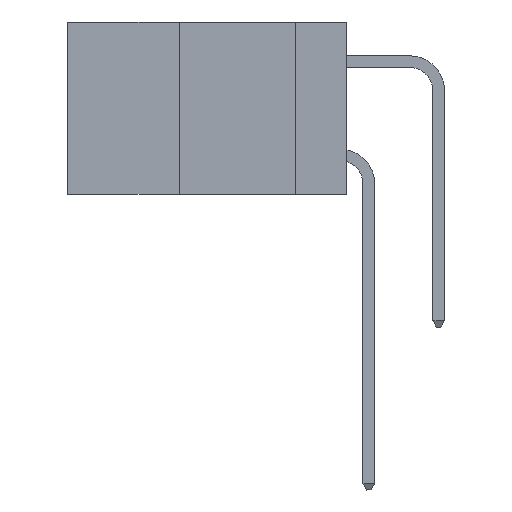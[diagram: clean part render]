
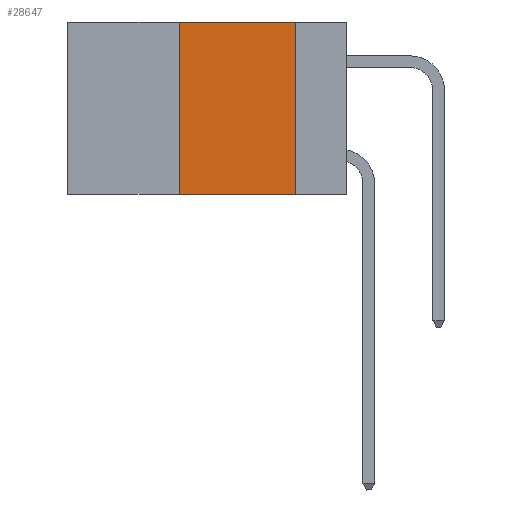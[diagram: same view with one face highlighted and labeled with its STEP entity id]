
A CAD part, left-side view. The second image highlights one B-rep face of the part: STEP entity #28647.
In plain terms, the highlighted planar face has unit normal (-1, 0, 0).
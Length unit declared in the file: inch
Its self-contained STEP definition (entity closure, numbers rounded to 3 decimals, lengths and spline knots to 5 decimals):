
#821 = CARTESIAN_POINT ( 'NONE',  ( 0., 0.11, -0.37 ) ) ;
#1053 = CARTESIAN_POINT ( 'NONE',  ( 0., 0.6, 0. ) ) ;
#2817 = DIRECTION ( 'NONE',  ( 0., 0., -1. ) ) ;
#2884 = CARTESIAN_POINT ( 'NONE',  ( 0., 0.36, -0.37 ) ) ;
#3447 = LINE ( 'NONE', #1053, #16288 ) ;
#3951 = EDGE_CURVE ( 'NONE', #26506, #30166, #3447, .T. ) ;
#4082 = CARTESIAN_POINT ( 'NONE',  ( 0., 0.11, 0. ) ) ;
#5867 = CARTESIAN_POINT ( 'NONE',  ( 0., 0.6, -0.37 ) ) ;
#6310 = VECTOR ( 'NONE', #28611, 39.37008 ) ;
#7259 = VECTOR ( 'NONE', #16170, 39.37008 ) ;
#8725 = DIRECTION ( 'NONE',  ( 0., -1., 0. ) ) ;
#8950 = FACE_OUTER_BOUND ( 'NONE', #31465, .T. ) ;
#9044 = ORIENTED_EDGE ( 'NONE', *, *, #19641, .F. ) ;
#10491 = PLANE ( 'NONE',  #29067 ) ;
#13149 = LINE ( 'NONE', #18684, #6310 ) ;
#16170 = DIRECTION ( 'NONE',  ( 0., -1., 0. ) ) ;
#16288 = VECTOR ( 'NONE', #8725, 39.37008 ) ;
#18013 = LINE ( 'NONE', #27522, #23905 ) ;
#18153 = DIRECTION ( 'NONE',  ( 1., 0., 0. ) ) ;
#18361 = VERTEX_POINT ( 'NONE', #2884 ) ;
#18684 = CARTESIAN_POINT ( 'NONE',  ( 0., 0.36, 0. ) ) ;
#19142 = ORIENTED_EDGE ( 'NONE', *, *, #3951, .F. ) ;
#19641 = EDGE_CURVE ( 'NONE', #18361, #26506, #13149, .T. ) ;
#20235 = ORIENTED_EDGE ( 'NONE', *, *, #26341, .F. ) ;
#20959 = CARTESIAN_POINT ( 'NONE',  ( 0., 0.36, 0. ) ) ;
#23143 = LINE ( 'NONE', #5867, #7259 ) ;
#23905 = VECTOR ( 'NONE', #27431, 39.37008 ) ;
#25301 = EDGE_CURVE ( 'NONE', #18361, #31702, #23143, .T. ) ;
#25613 = CARTESIAN_POINT ( 'NONE',  ( 0., 0.6, 0. ) ) ;
#26341 = EDGE_CURVE ( 'NONE', #30166, #31702, #18013, .T. ) ;
#26506 = VERTEX_POINT ( 'NONE', #20959 ) ;
#27431 = DIRECTION ( 'NONE',  ( 0., 0., -1. ) ) ;
#27522 = CARTESIAN_POINT ( 'NONE',  ( 0., 0.11, 0. ) ) ;
#28611 = DIRECTION ( 'NONE',  ( 0., 0., 1. ) ) ;
#28647 = ADVANCED_FACE ( 'NONE', ( #8950 ), #10491, .F. ) ;
#29067 = AXIS2_PLACEMENT_3D ( 'NONE', #25613, #18153, #2817 ) ;
#30166 = VERTEX_POINT ( 'NONE', #4082 ) ;
#30352 = ORIENTED_EDGE ( 'NONE', *, *, #25301, .T. ) ;
#31465 = EDGE_LOOP ( 'NONE', ( #20235, #19142, #9044, #30352 ) ) ;
#31702 = VERTEX_POINT ( 'NONE', #821 ) ;
